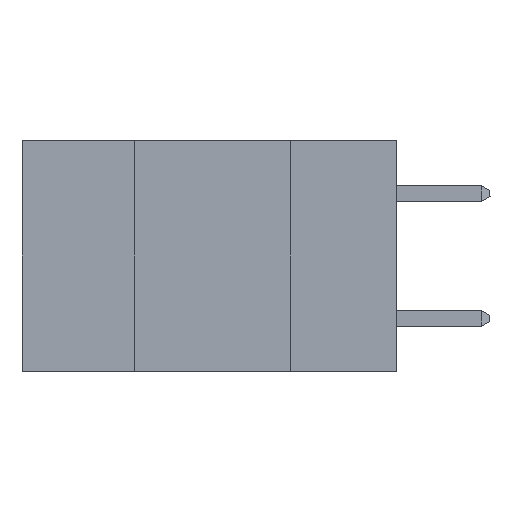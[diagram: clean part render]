
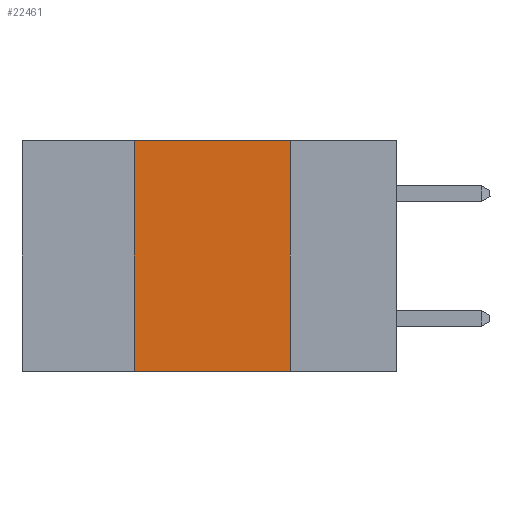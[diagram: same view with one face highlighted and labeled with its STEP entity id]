
A CAD part, left-side view. The second image highlights one B-rep face of the part: STEP entity #22461.
In plain terms, the highlighted planar face has unit normal (-1, 0, 0).
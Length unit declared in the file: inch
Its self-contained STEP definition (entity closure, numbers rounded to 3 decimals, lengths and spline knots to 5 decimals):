
#732 = EDGE_CURVE ( 'NONE', #13958, #15517, #15301, .T. ) ;
#754 = FACE_OUTER_BOUND ( 'NONE', #26213, .T. ) ;
#1212 = CARTESIAN_POINT ( 'NONE',  ( 0., 0.42, -0.37 ) ) ;
#3142 = LINE ( 'NONE', #13883, #17034 ) ;
#4748 = CARTESIAN_POINT ( 'NONE',  ( 0., 0.42, 0. ) ) ;
#5151 = CARTESIAN_POINT ( 'NONE',  ( 0., 0.6, 0. ) ) ;
#5953 = EDGE_CURVE ( 'NONE', #13958, #21953, #20237, .T. ) ;
#7172 = DIRECTION ( 'NONE',  ( 0., -1., 0. ) ) ;
#8542 = EDGE_CURVE ( 'NONE', #16852, #21953, #3142, .T. ) ;
#10138 = VECTOR ( 'NONE', #20335, 39.37008 ) ;
#10700 = DIRECTION ( 'NONE',  ( 1., 0., 0. ) ) ;
#11032 = CARTESIAN_POINT ( 'NONE',  ( 0., 0.6, -0.37 ) ) ;
#13405 = CARTESIAN_POINT ( 'NONE',  ( 0., 0.42, 0. ) ) ;
#13883 = CARTESIAN_POINT ( 'NONE',  ( 0., 0.17, 0. ) ) ;
#13958 = VERTEX_POINT ( 'NONE', #1212 ) ;
#14648 = VECTOR ( 'NONE', #17811, 39.37008 ) ;
#15095 = PLANE ( 'NONE',  #28014 ) ;
#15301 = LINE ( 'NONE', #4748, #14648 ) ;
#15517 = VERTEX_POINT ( 'NONE', #13405 ) ;
#16005 = ORIENTED_EDGE ( 'NONE', *, *, #732, .F. ) ;
#16852 = VERTEX_POINT ( 'NONE', #17459 ) ;
#17034 = VECTOR ( 'NONE', #22606, 39.37008 ) ;
#17459 = CARTESIAN_POINT ( 'NONE',  ( 0., 0.17, 0. ) ) ;
#17811 = DIRECTION ( 'NONE',  ( 0., 0., 1. ) ) ;
#20237 = LINE ( 'NONE', #11032, #25326 ) ;
#20335 = DIRECTION ( 'NONE',  ( 0., -1., 0. ) ) ;
#20688 = ORIENTED_EDGE ( 'NONE', *, *, #5953, .T. ) ;
#20996 = ORIENTED_EDGE ( 'NONE', *, *, #24388, .F. ) ;
#21040 = LINE ( 'NONE', #5151, #10138 ) ;
#21553 = DIRECTION ( 'NONE',  ( 0., 0., -1. ) ) ;
#21869 = ORIENTED_EDGE ( 'NONE', *, *, #8542, .F. ) ;
#21953 = VERTEX_POINT ( 'NONE', #21969 ) ;
#21969 = CARTESIAN_POINT ( 'NONE',  ( 0., 0.17, -0.37 ) ) ;
#22461 = ADVANCED_FACE ( 'NONE', ( #754 ), #15095, .F. ) ;
#22606 = DIRECTION ( 'NONE',  ( 0., 0., -1. ) ) ;
#24388 = EDGE_CURVE ( 'NONE', #15517, #16852, #21040, .T. ) ;
#25326 = VECTOR ( 'NONE', #7172, 39.37008 ) ;
#26213 = EDGE_LOOP ( 'NONE', ( #21869, #20996, #16005, #20688 ) ) ;
#27946 = CARTESIAN_POINT ( 'NONE',  ( 0., 0.6, 0. ) ) ;
#28014 = AXIS2_PLACEMENT_3D ( 'NONE', #27946, #10700, #21553 ) ;
